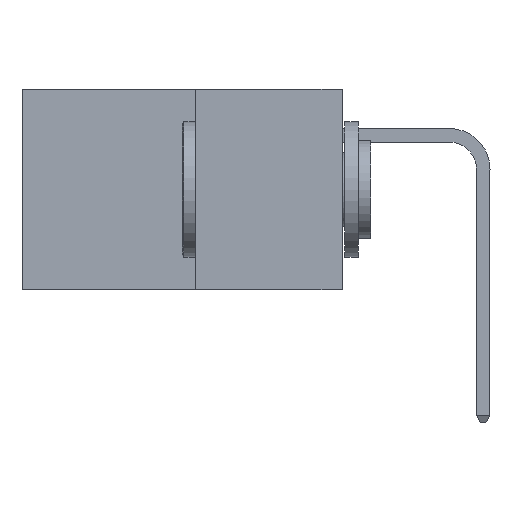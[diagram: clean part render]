
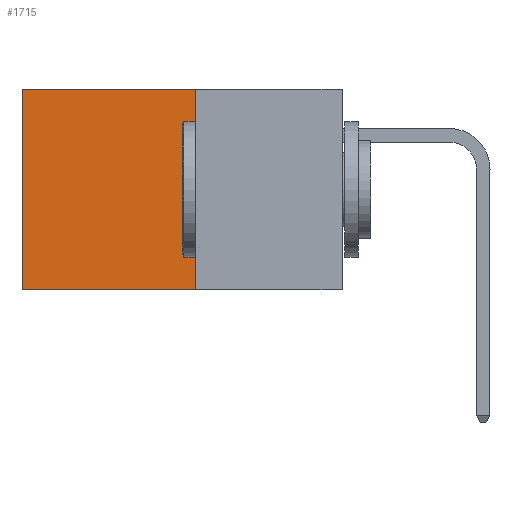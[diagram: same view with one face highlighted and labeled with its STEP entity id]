
A CAD part, left-side view. The second image highlights one B-rep face of the part: STEP entity #1715.
In plain terms, the highlighted planar face has unit normal (-1, 0, 0).
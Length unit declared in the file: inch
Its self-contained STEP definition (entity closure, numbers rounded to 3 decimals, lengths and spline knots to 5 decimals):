
#12 = VERTEX_POINT ( 'NONE', #50 ) ;
#50 = CARTESIAN_POINT ( 'NONE',  ( 0.277, 0.27, 0. ) ) ;
#668 = VECTOR ( 'NONE', #15125, 39.37008 ) ;
#1293 = EDGE_CURVE ( 'NONE', #11812, #5232, #13130, .T. ) ;
#1715 = ADVANCED_FACE ( 'NONE', ( #11557 ), #2001, .F. ) ;
#1934 = VERTEX_POINT ( 'NONE', #5835 ) ;
#2001 = PLANE ( 'NONE',  #11657 ) ;
#2255 = LINE ( 'NONE', #7230, #16786 ) ;
#2723 = EDGE_CURVE ( 'NONE', #12, #11812, #2255, .T. ) ;
#3300 = DIRECTION ( 'NONE',  ( 0., 0., -1. ) ) ;
#3303 = CARTESIAN_POINT ( 'NONE',  ( 0.277, 0.59, -0.37 ) ) ;
#5232 = VERTEX_POINT ( 'NONE', #3303 ) ;
#5835 = CARTESIAN_POINT ( 'NONE',  ( 0.277, 0.59, 0. ) ) ;
#6976 = CARTESIAN_POINT ( 'NONE',  ( 0.277, 0.27, 0. ) ) ;
#7099 = EDGE_LOOP ( 'NONE', ( #9638, #9433, #11671, #17328 ) ) ;
#7116 = CARTESIAN_POINT ( 'NONE',  ( 0.277, 0.27, -0.37 ) ) ;
#7230 = CARTESIAN_POINT ( 'NONE',  ( 0.277, 0.27, -0.37 ) ) ;
#8854 = CARTESIAN_POINT ( 'NONE',  ( 0.277, 0.27, -0.37 ) ) ;
#9280 = LINE ( 'NONE', #6976, #15859 ) ;
#9433 = ORIENTED_EDGE ( 'NONE', *, *, #1293, .F. ) ;
#9638 = ORIENTED_EDGE ( 'NONE', *, *, #13624, .T. ) ;
#10768 = DIRECTION ( 'NONE',  ( 0., 0., -1. ) ) ;
#11511 = LINE ( 'NONE', #13717, #668 ) ;
#11557 = FACE_OUTER_BOUND ( 'NONE', #7099, .T. ) ;
#11657 = AXIS2_PLACEMENT_3D ( 'NONE', #7116, #14424, #3300 ) ;
#11671 = ORIENTED_EDGE ( 'NONE', *, *, #2723, .F. ) ;
#11812 = VERTEX_POINT ( 'NONE', #15296 ) ;
#13130 = LINE ( 'NONE', #8854, #16365 ) ;
#13624 = EDGE_CURVE ( 'NONE', #1934, #5232, #11511, .T. ) ;
#13717 = CARTESIAN_POINT ( 'NONE',  ( 0.277, 0.59, -0.37 ) ) ;
#13775 = EDGE_CURVE ( 'NONE', #12, #1934, #9280, .T. ) ;
#14017 = DIRECTION ( 'NONE',  ( 0., 1., 0. ) ) ;
#14424 = DIRECTION ( 'NONE',  ( 1., 0., 0. ) ) ;
#15125 = DIRECTION ( 'NONE',  ( 0., 0., -1. ) ) ;
#15296 = CARTESIAN_POINT ( 'NONE',  ( 0.277, 0.27, -0.37 ) ) ;
#15859 = VECTOR ( 'NONE', #14017, 39.37008 ) ;
#16365 = VECTOR ( 'NONE', #17332, 39.37008 ) ;
#16786 = VECTOR ( 'NONE', #10768, 39.37008 ) ;
#17328 = ORIENTED_EDGE ( 'NONE', *, *, #13775, .T. ) ;
#17332 = DIRECTION ( 'NONE',  ( 0., 1., 0. ) ) ;
